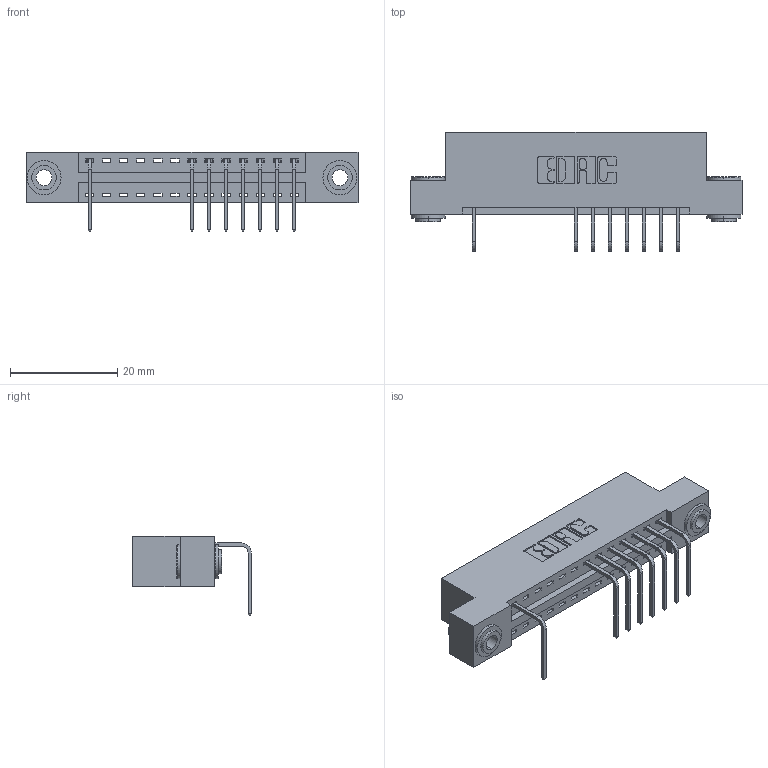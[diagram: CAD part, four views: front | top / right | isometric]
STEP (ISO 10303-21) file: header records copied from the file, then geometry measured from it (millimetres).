
FILE_DESCRIPTION (( 'STEP AP203' ), '1' );
FILE_NAME ('346-013-558-103.STEP', '2018-08-20T00:03:46', ( '' ), ( '' ), 'SwSTEP 2.0', 'SolidWorks 2016', '' );
FILE_SCHEMA (( 'CONFIG_CONTROL_DESIGN' ));
Length unit declared in the file: inch
Products named in the file (4): 346-013-558-103; 346 Part_Flush Mounting Lugs - 0.156 Dia-TH; 345-292-001_558 Tail - 2; 345-250-002_345-250-002-102
Assembly tree (11 placements, depth 2):
  346-013-558-103
    346 Part_Flush Mounting Lugs - 0.156 Dia-TH
    345-292-001_558 Tail - 2  x8
    345-250-002_345-250-002-102  x2
Bounding box: 61.85 x 22.16 x 14.73 mm (x, y, z)
Volume: 5709.4 mm3; surface area: 6893.6 mm2
Topology: 11 solids, 11 shells, 700 faces, 2071 edges, 1366 vertices
Faces by surface type: plane 472, cylinder 220, cone 8
Entity records: 12546 total; most frequent: CARTESIAN_POINT 2161, ORIENTED_EDGE 2106, DIRECTION 1967, EDGE_CURVE 1053, VECTOR 845, LINE 845, VERTEX_POINT 698, AXIS2_PLACEMENT_3D 561
